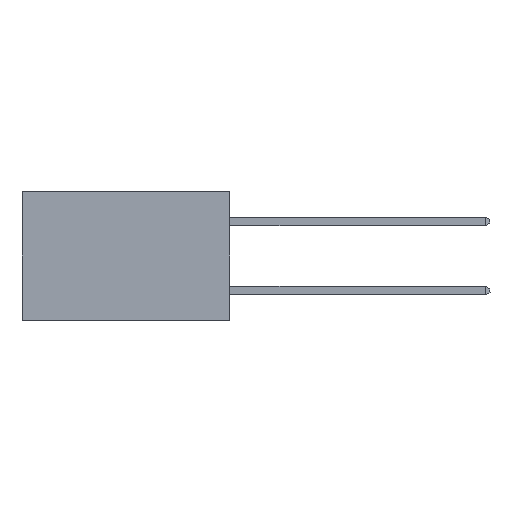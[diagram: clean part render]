
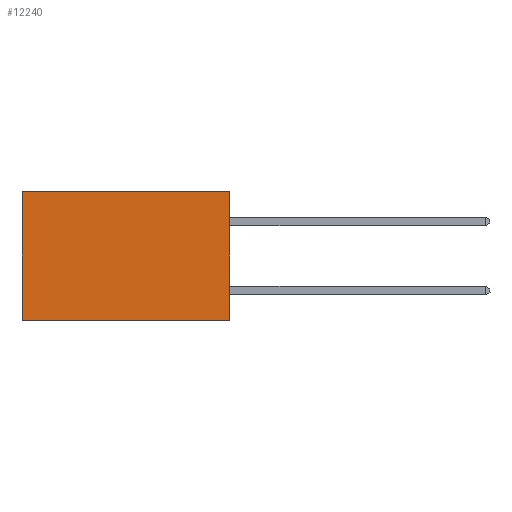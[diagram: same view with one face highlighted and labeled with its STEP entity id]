
A CAD part, left-side view. The second image highlights one B-rep face of the part: STEP entity #12240.
In plain terms, the highlighted planar face has unit normal (-1, 0, 0).
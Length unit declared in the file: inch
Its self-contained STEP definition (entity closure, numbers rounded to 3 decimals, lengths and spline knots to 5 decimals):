
#1208 = CARTESIAN_POINT ( 'NONE',  ( 0.298, 0., -0.37 ) ) ;
#1598 = VERTEX_POINT ( 'NONE', #9265 ) ;
#1730 = EDGE_LOOP ( 'NONE', ( #11933, #20441, #10315, #5683 ) ) ;
#2111 = DIRECTION ( 'NONE',  ( 0., 0., -1. ) ) ;
#2169 = LINE ( 'NONE', #16826, #14193 ) ;
#3082 = EDGE_CURVE ( 'NONE', #12386, #7642, #17648, .T. ) ;
#4543 = CARTESIAN_POINT ( 'NONE',  ( 0.298, 0., -0.37 ) ) ;
#4749 = VECTOR ( 'NONE', #2111, 39.37008 ) ;
#4841 = AXIS2_PLACEMENT_3D ( 'NONE', #9375, #9172, #7496 ) ;
#4898 = CARTESIAN_POINT ( 'NONE',  ( 0.298, 0., 0. ) ) ;
#5683 = ORIENTED_EDGE ( 'NONE', *, *, #9624, .T. ) ;
#6141 = EDGE_CURVE ( 'NONE', #1598, #7642, #9888, .T. ) ;
#7370 = EDGE_CURVE ( 'NONE', #17602, #12386, #2169, .T. ) ;
#7496 = DIRECTION ( 'NONE',  ( 0., 0., -1. ) ) ;
#7642 = VERTEX_POINT ( 'NONE', #20242 ) ;
#8766 = DIRECTION ( 'NONE',  ( 0., 0., -1. ) ) ;
#9172 = DIRECTION ( 'NONE',  ( 1., 0., 0. ) ) ;
#9265 = CARTESIAN_POINT ( 'NONE',  ( 0.298, 0.6, 0. ) ) ;
#9375 = CARTESIAN_POINT ( 'NONE',  ( 0.298, 0., 0. ) ) ;
#9624 = EDGE_CURVE ( 'NONE', #17602, #1598, #10512, .T. ) ;
#9851 = DIRECTION ( 'NONE',  ( 0., 1., 0. ) ) ;
#9888 = LINE ( 'NONE', #16651, #4749 ) ;
#10315 = ORIENTED_EDGE ( 'NONE', *, *, #7370, .F. ) ;
#10415 = CARTESIAN_POINT ( 'NONE',  ( 0.298, 0., 0. ) ) ;
#10512 = LINE ( 'NONE', #4898, #20161 ) ;
#10758 = PLANE ( 'NONE',  #4841 ) ;
#11333 = VECTOR ( 'NONE', #19237, 39.37008 ) ;
#11933 = ORIENTED_EDGE ( 'NONE', *, *, #6141, .T. ) ;
#12203 = FACE_OUTER_BOUND ( 'NONE', #1730, .T. ) ;
#12240 = ADVANCED_FACE ( 'NONE', ( #12203 ), #10758, .F. ) ;
#12386 = VERTEX_POINT ( 'NONE', #4543 ) ;
#14193 = VECTOR ( 'NONE', #8766, 39.37008 ) ;
#16651 = CARTESIAN_POINT ( 'NONE',  ( 0.298, 0.6, 0. ) ) ;
#16826 = CARTESIAN_POINT ( 'NONE',  ( 0.298, 0., 0. ) ) ;
#17602 = VERTEX_POINT ( 'NONE', #10415 ) ;
#17648 = LINE ( 'NONE', #1208, #11333 ) ;
#19237 = DIRECTION ( 'NONE',  ( 0., 1., 0. ) ) ;
#20161 = VECTOR ( 'NONE', #9851, 39.37008 ) ;
#20242 = CARTESIAN_POINT ( 'NONE',  ( 0.298, 0.6, -0.37 ) ) ;
#20441 = ORIENTED_EDGE ( 'NONE', *, *, #3082, .F. ) ;
